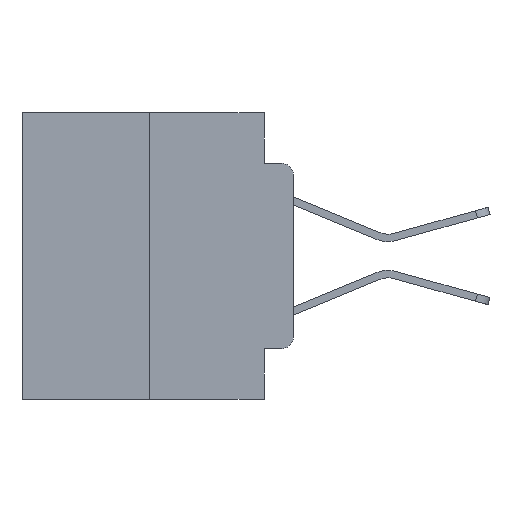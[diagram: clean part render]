
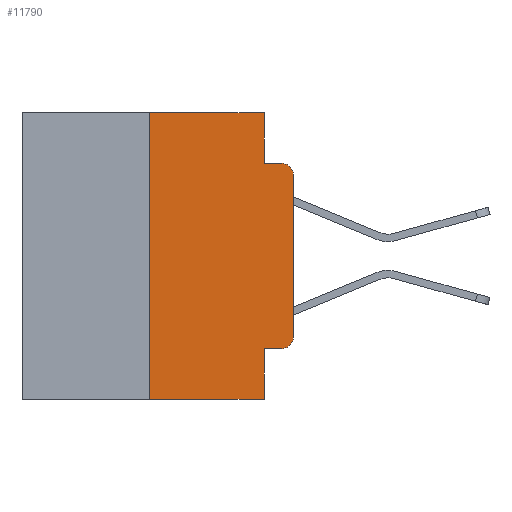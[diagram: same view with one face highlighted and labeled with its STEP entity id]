
A CAD part, left-side view. The second image highlights one B-rep face of the part: STEP entity #11790.
In plain terms, the highlighted planar face has unit normal (-1, 0, 0).
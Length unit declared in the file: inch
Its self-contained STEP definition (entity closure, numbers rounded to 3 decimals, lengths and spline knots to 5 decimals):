
#35 = VECTOR ( 'NONE', #25361, 39.37008 ) ;
#432 = DIRECTION ( 'NONE',  ( 0., 0., -1. ) ) ;
#532 = VECTOR ( 'NONE', #22599, 39.37008 ) ;
#1365 = VERTEX_POINT ( 'NONE', #16116 ) ;
#1432 = ORIENTED_EDGE ( 'NONE', *, *, #24058, .T. ) ;
#1530 = DIRECTION ( 'NONE',  ( 0., 0., -1. ) ) ;
#1645 = LINE ( 'NONE', #12636, #7571 ) ;
#1952 = LINE ( 'NONE', #3849, #532 ) ;
#2203 = CARTESIAN_POINT ( 'NONE',  ( 0., 0.051, -0.4115 ) ) ;
#2934 = CIRCLE ( 'NONE', #18992, 0.02 ) ;
#2939 = CARTESIAN_POINT ( 'NONE',  ( 0., 0.051, -0.4115 ) ) ;
#3166 = VERTEX_POINT ( 'NONE', #2939 ) ;
#3849 = CARTESIAN_POINT ( 'NONE',  ( 0., 0.473, 0. ) ) ;
#5103 = EDGE_CURVE ( 'NONE', #13807, #1365, #1952, .T. ) ;
#5838 = CARTESIAN_POINT ( 'NONE',  ( 0., 0., 0. ) ) ;
#5982 = ORIENTED_EDGE ( 'NONE', *, *, #5103, .F. ) ;
#6204 = VERTEX_POINT ( 'NONE', #18195 ) ;
#6275 = EDGE_CURVE ( 'NONE', #18521, #26348, #2934, .T. ) ;
#6489 = DIRECTION ( 'NONE',  ( -1., 0., 0. ) ) ;
#7371 = ORIENTED_EDGE ( 'NONE', *, *, #9159, .F. ) ;
#7571 = VECTOR ( 'NONE', #14704, 39.37008 ) ;
#7743 = VERTEX_POINT ( 'NONE', #27058 ) ;
#7746 = EDGE_CURVE ( 'NONE', #3166, #18521, #12650, .T. ) ;
#7995 = CARTESIAN_POINT ( 'NONE',  ( 0., 0., -0.1085 ) ) ;
#8349 = ORIENTED_EDGE ( 'NONE', *, *, #21513, .T. ) ;
#8360 = FACE_OUTER_BOUND ( 'NONE', #16882, .T. ) ;
#8831 = DIRECTION ( 'NONE',  ( 0., -1., 0. ) ) ;
#9159 = EDGE_CURVE ( 'NONE', #3166, #23522, #26808, .T. ) ;
#9254 = LINE ( 'NONE', #20156, #24905 ) ;
#10384 = PLANE ( 'NONE',  #16701 ) ;
#10573 = VECTOR ( 'NONE', #432, 39.37008 ) ;
#10934 = DIRECTION ( 'NONE',  ( 0., 0., 1. ) ) ;
#11336 = VECTOR ( 'NONE', #8831, 39.37008 ) ;
#11739 = VERTEX_POINT ( 'NONE', #26583 ) ;
#11790 = ADVANCED_FACE ( 'NONE', ( #8360 ), #10384, .F. ) ;
#11941 = EDGE_CURVE ( 'NONE', #7743, #13807, #20879, .T. ) ;
#12604 = DIRECTION ( 'NONE',  ( 1., 0., 0. ) ) ;
#12636 = CARTESIAN_POINT ( 'NONE',  ( 0., 0.051, -0.0885 ) ) ;
#12650 = LINE ( 'NONE', #2203, #11336 ) ;
#12935 = ORIENTED_EDGE ( 'NONE', *, *, #7746, .T. ) ;
#13361 = EDGE_CURVE ( 'NONE', #1365, #11739, #9254, .T. ) ;
#13517 = CARTESIAN_POINT ( 'NONE',  ( 0., 0.051, -0.5 ) ) ;
#13620 = AXIS2_PLACEMENT_3D ( 'NONE', #18882, #6489, #20941 ) ;
#13807 = VERTEX_POINT ( 'NONE', #25710 ) ;
#13892 = ORIENTED_EDGE ( 'NONE', *, *, #18775, .T. ) ;
#14391 = DIRECTION ( 'NONE',  ( -1., 0., 0. ) ) ;
#14704 = DIRECTION ( 'NONE',  ( 0., -1., 0. ) ) ;
#14714 = EDGE_CURVE ( 'NONE', #11739, #6204, #1645, .T. ) ;
#15035 = CARTESIAN_POINT ( 'NONE',  ( 0., 0.25, 0. ) ) ;
#15478 = VECTOR ( 'NONE', #10934, 39.37008 ) ;
#15926 = VECTOR ( 'NONE', #18280, 39.37008 ) ;
#16116 = CARTESIAN_POINT ( 'NONE',  ( 0., 0.051, 0. ) ) ;
#16423 = LINE ( 'NONE', #19330, #35 ) ;
#16600 = CARTESIAN_POINT ( 'NONE',  ( 0., 0.473, 0. ) ) ;
#16701 = AXIS2_PLACEMENT_3D ( 'NONE', #16600, #12604, #26754 ) ;
#16882 = EDGE_LOOP ( 'NONE', ( #8349, #13892, #20548, #21203, #5982, #22457, #1432, #7371, #12935, #18965 ) ) ;
#17104 = CARTESIAN_POINT ( 'NONE',  ( 0., 0., -0.3915 ) ) ;
#18195 = CARTESIAN_POINT ( 'NONE',  ( 0., 0.02, -0.0885 ) ) ;
#18199 = DIRECTION ( 'NONE',  ( 0., 0., -1. ) ) ;
#18280 = DIRECTION ( 'NONE',  ( 0., 0., 1. ) ) ;
#18521 = VERTEX_POINT ( 'NONE', #20042 ) ;
#18775 = EDGE_CURVE ( 'NONE', #22458, #6204, #21754, .T. ) ;
#18882 = CARTESIAN_POINT ( 'NONE',  ( 0., 0.02, -0.1085 ) ) ;
#18965 = ORIENTED_EDGE ( 'NONE', *, *, #6275, .T. ) ;
#18992 = AXIS2_PLACEMENT_3D ( 'NONE', #26483, #14391, #1530 ) ;
#19330 = CARTESIAN_POINT ( 'NONE',  ( 0., 0.473, -0.5 ) ) ;
#20042 = CARTESIAN_POINT ( 'NONE',  ( 0., 0.02, -0.4115 ) ) ;
#20156 = CARTESIAN_POINT ( 'NONE',  ( 0., 0.051, 0. ) ) ;
#20548 = ORIENTED_EDGE ( 'NONE', *, *, #14714, .F. ) ;
#20879 = LINE ( 'NONE', #15035, #15478 ) ;
#20941 = DIRECTION ( 'NONE',  ( 0., 0., -1. ) ) ;
#21203 = ORIENTED_EDGE ( 'NONE', *, *, #13361, .F. ) ;
#21352 = LINE ( 'NONE', #5838, #15926 ) ;
#21513 = EDGE_CURVE ( 'NONE', #26348, #22458, #21352, .T. ) ;
#21754 = CIRCLE ( 'NONE', #13620, 0.02 ) ;
#22457 = ORIENTED_EDGE ( 'NONE', *, *, #11941, .F. ) ;
#22458 = VERTEX_POINT ( 'NONE', #7995 ) ;
#22599 = DIRECTION ( 'NONE',  ( 0., -1., 0. ) ) ;
#23522 = VERTEX_POINT ( 'NONE', #13517 ) ;
#24058 = EDGE_CURVE ( 'NONE', #7743, #23522, #16423, .T. ) ;
#24905 = VECTOR ( 'NONE', #18199, 39.37008 ) ;
#25361 = DIRECTION ( 'NONE',  ( 0., -1., 0. ) ) ;
#25531 = CARTESIAN_POINT ( 'NONE',  ( 0., 0.051, 0. ) ) ;
#25710 = CARTESIAN_POINT ( 'NONE',  ( 0., 0.25, 0. ) ) ;
#26348 = VERTEX_POINT ( 'NONE', #17104 ) ;
#26483 = CARTESIAN_POINT ( 'NONE',  ( 0., 0.02, -0.3915 ) ) ;
#26583 = CARTESIAN_POINT ( 'NONE',  ( 0., 0.051, -0.0885 ) ) ;
#26754 = DIRECTION ( 'NONE',  ( 0., 0., -1. ) ) ;
#26808 = LINE ( 'NONE', #25531, #10573 ) ;
#27058 = CARTESIAN_POINT ( 'NONE',  ( 0., 0.25, -0.5 ) ) ;
